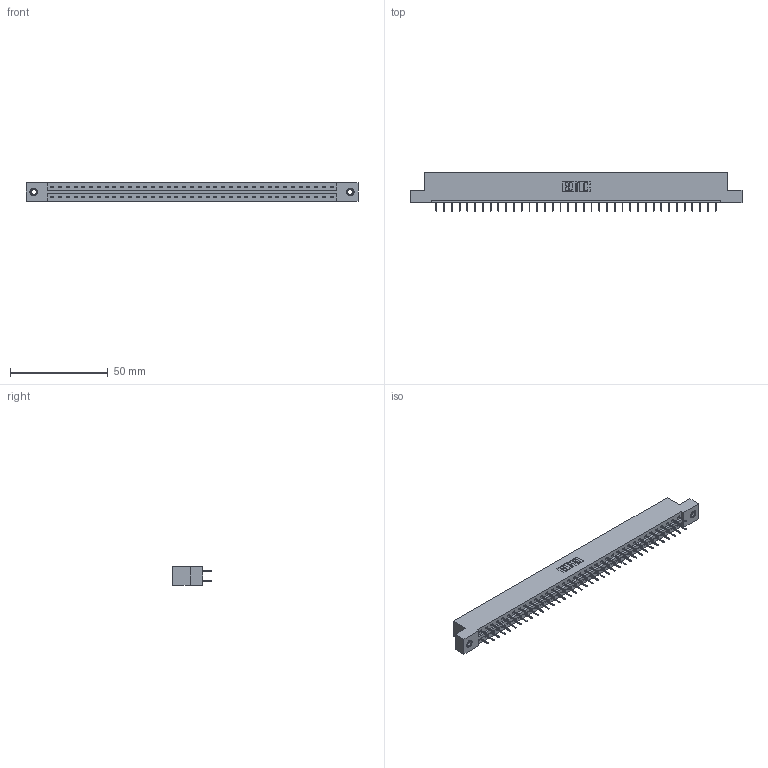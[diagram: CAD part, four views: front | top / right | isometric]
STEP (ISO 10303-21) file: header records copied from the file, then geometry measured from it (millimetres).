
FILE_DESCRIPTION (( 'STEP AP203' ), '1' );
FILE_NAME ('387-074-524-207.STEP', '2019-10-22T01:26:23', ( '' ), ( '' ), 'SwSTEP 2.0', 'SolidWorks 2016', '' );
FILE_SCHEMA (( 'CONFIG_CONTROL_DESIGN' ));
Length unit declared in the file: inch
Products named in the file (4): 387-074-524-207; 345-292-001_345-293-124; 337 Part_Flush Mounting Lugs - 0.156 Dia-TI; 345-250-001_345-250-005-103
Assembly tree (77 placements, depth 2):
  387-074-524-207
    337 Part_Flush Mounting Lugs - 0.156 Dia-TI
    345-292-001_345-293-124  x74
    345-250-001_345-250-005-103  x2
Bounding box: 169.62 x 19.69 x 9.4 mm (x, y, z)
Volume: 17684 mm3; surface area: 19632.3 mm2
Topology: 77 solids, 77 shells, 4466 faces, 12657 edges, 8134 vertices
Faces by surface type: plane 3358, cylinder 1092, cone 12, torus 4
Entity records: 30594 total; most frequent: CARTESIAN_POINT 5137, ORIENTED_EDGE 5066, DIRECTION 4411, EDGE_CURVE 2533, VECTOR 2389, LINE 2389, VERTEX_POINT 1680, AXIS2_PLACEMENT_3D 1011
